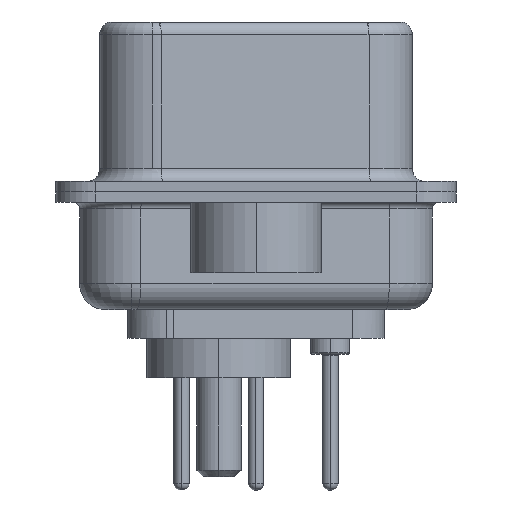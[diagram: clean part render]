
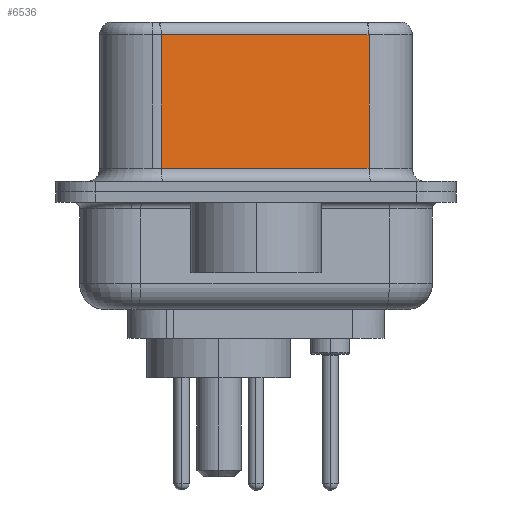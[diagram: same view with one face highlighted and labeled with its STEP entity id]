
A CAD part, left-side view. The second image highlights one B-rep face of the part: STEP entity #6536.
In plain terms, the highlighted planar face has unit normal (-0.985, -0.174, 0).
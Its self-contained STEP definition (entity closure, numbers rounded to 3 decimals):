
#33 = ORIENTED_EDGE ( 'NONE', *, *, #15771, .T. ) ;
#467 = LINE ( 'NONE', #25376, #21424 ) ;
#1267 = CARTESIAN_POINT ( 'NONE',  ( 5.132, -4.322, 6.02 ) ) ;
#2880 = LINE ( 'NONE', #21767, #23807 ) ;
#3102 = CARTESIAN_POINT ( 'NONE',  ( 5.132, -4.322, 6.52 ) ) ;
#3379 = ORIENTED_EDGE ( 'NONE', *, *, #23399, .T. ) ;
#3423 = EDGE_LOOP ( 'NONE', ( #24517, #33, #3379, #14773 ) ) ;
#4522 = VERTEX_POINT ( 'NONE', #17020 ) ;
#4528 = VECTOR ( 'NONE', #14791, 1000. ) ;
#6536 = ADVANCED_FACE ( 'NONE', ( #17143 ), #7499, .F. ) ;
#6983 = EDGE_CURVE ( 'NONE', #15807, #4522, #2880, .T. ) ;
#7499 = PLANE ( 'NONE',  #13579 ) ;
#9195 = VERTEX_POINT ( 'NONE', #10555 ) ;
#9869 = LINE ( 'NONE', #16756, #4528 ) ;
#10555 = CARTESIAN_POINT ( 'NONE',  ( 5.132, -4.322, 6.02 ) ) ;
#11689 = CARTESIAN_POINT ( 'NONE',  ( 3.73, 3.628, 6.02 ) ) ;
#12546 = VECTOR ( 'NONE', #13372, 1000. ) ;
#13196 = DIRECTION ( 'NONE',  ( 0., 0., -1. ) ) ;
#13372 = DIRECTION ( 'NONE',  ( -0.174, 0.985, 0. ) ) ;
#13579 = AXIS2_PLACEMENT_3D ( 'NONE', #3102, #19349, #19286 ) ;
#13798 = LINE ( 'NONE', #1267, #12546 ) ;
#14707 = VERTEX_POINT ( 'NONE', #11689 ) ;
#14773 = ORIENTED_EDGE ( 'NONE', *, *, #6983, .T. ) ;
#14791 = DIRECTION ( 'NONE',  ( 0., 0., -1. ) ) ;
#15771 = EDGE_CURVE ( 'NONE', #9195, #14707, #13798, .T. ) ;
#15807 = VERTEX_POINT ( 'NONE', #21653 ) ;
#16076 = DIRECTION ( 'NONE',  ( 0.174, -0.985, 0. ) ) ;
#16756 = CARTESIAN_POINT ( 'NONE',  ( 5.132, -4.322, 6.52 ) ) ;
#17020 = CARTESIAN_POINT ( 'NONE',  ( 5.132, -4.322, 0.9 ) ) ;
#17143 = FACE_OUTER_BOUND ( 'NONE', #3423, .T. ) ;
#19262 = EDGE_CURVE ( 'NONE', #9195, #4522, #9869, .T. ) ;
#19286 = DIRECTION ( 'NONE',  ( -0.174, 0.985, 0. ) ) ;
#19349 = DIRECTION ( 'NONE',  ( 0.985, 0.174, 0. ) ) ;
#21424 = VECTOR ( 'NONE', #13196, 1000. ) ;
#21653 = CARTESIAN_POINT ( 'NONE',  ( 3.73, 3.628, 0.9 ) ) ;
#21767 = CARTESIAN_POINT ( 'NONE',  ( 5.132, -4.322, 0.9 ) ) ;
#23399 = EDGE_CURVE ( 'NONE', #14707, #15807, #467, .T. ) ;
#23807 = VECTOR ( 'NONE', #16076, 1000. ) ;
#24517 = ORIENTED_EDGE ( 'NONE', *, *, #19262, .F. ) ;
#25376 = CARTESIAN_POINT ( 'NONE',  ( 3.73, 3.628, 6.52 ) ) ;
